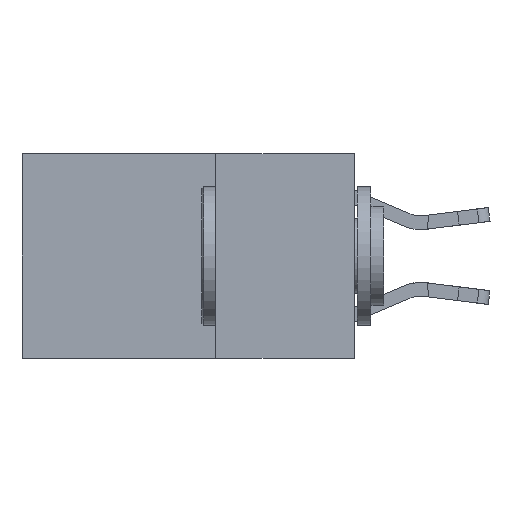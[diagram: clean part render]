
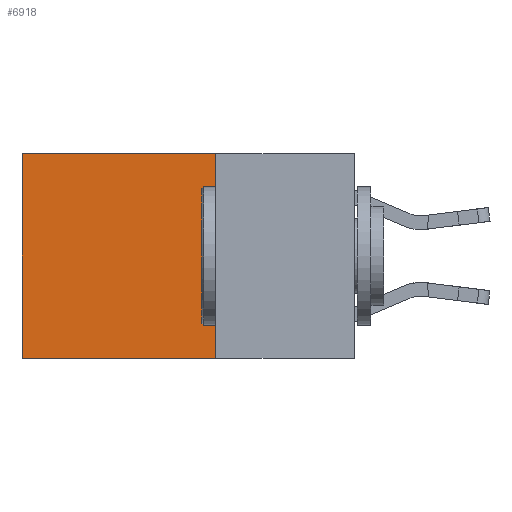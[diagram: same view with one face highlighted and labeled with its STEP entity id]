
A CAD part, left-side view. The second image highlights one B-rep face of the part: STEP entity #6918.
In plain terms, the highlighted planar face has unit normal (-1, 0, 0).
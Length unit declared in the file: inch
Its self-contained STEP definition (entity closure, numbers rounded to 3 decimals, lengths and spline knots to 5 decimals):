
#25 = LINE ( 'NONE', #16670, #8484 ) ;
#30 = VERTEX_POINT ( 'NONE', #15405 ) ;
#818 = AXIS2_PLACEMENT_3D ( 'NONE', #14815, #3728, #6355 ) ;
#2178 = FACE_OUTER_BOUND ( 'NONE', #3629, .T. ) ;
#3294 = CARTESIAN_POINT ( 'NONE',  ( 0.2625, 0.6, 0. ) ) ;
#3479 = VECTOR ( 'NONE', #13571, 39.37008 ) ;
#3629 = EDGE_LOOP ( 'NONE', ( #8943, #17262, #16679, #10003 ) ) ;
#3728 = DIRECTION ( 'NONE',  ( 1., 0., 0. ) ) ;
#3860 = CARTESIAN_POINT ( 'NONE',  ( 0.2625, 0.25, 0. ) ) ;
#3932 = EDGE_CURVE ( 'NONE', #8075, #30, #25, .T. ) ;
#4221 = DIRECTION ( 'NONE',  ( 0., 0., -1. ) ) ;
#5716 = EDGE_CURVE ( 'NONE', #9379, #9397, #15033, .T. ) ;
#5931 = EDGE_CURVE ( 'NONE', #9379, #8075, #6485, .T. ) ;
#6355 = DIRECTION ( 'NONE',  ( 0., 0., -1. ) ) ;
#6485 = LINE ( 'NONE', #17642, #11206 ) ;
#6918 = ADVANCED_FACE ( 'NONE', ( #2178 ), #17601, .F. ) ;
#7273 = LINE ( 'NONE', #12744, #7653 ) ;
#7653 = VECTOR ( 'NONE', #12839, 39.37008 ) ;
#7852 = DIRECTION ( 'NONE',  ( 0., 1., 0. ) ) ;
#8075 = VERTEX_POINT ( 'NONE', #3294 ) ;
#8484 = VECTOR ( 'NONE', #4221, 39.37008 ) ;
#8943 = ORIENTED_EDGE ( 'NONE', *, *, #3932, .T. ) ;
#9379 = VERTEX_POINT ( 'NONE', #3860 ) ;
#9397 = VERTEX_POINT ( 'NONE', #11341 ) ;
#9933 = EDGE_CURVE ( 'NONE', #9397, #30, #7273, .T. ) ;
#10003 = ORIENTED_EDGE ( 'NONE', *, *, #5931, .T. ) ;
#11206 = VECTOR ( 'NONE', #7852, 39.37008 ) ;
#11341 = CARTESIAN_POINT ( 'NONE',  ( 0.2625, 0.25, -0.37 ) ) ;
#12744 = CARTESIAN_POINT ( 'NONE',  ( 0.2625, 0.25, -0.37 ) ) ;
#12839 = DIRECTION ( 'NONE',  ( 0., 1., 0. ) ) ;
#13571 = DIRECTION ( 'NONE',  ( 0., 0., -1. ) ) ;
#13766 = CARTESIAN_POINT ( 'NONE',  ( 0.2625, 0.25, 0. ) ) ;
#14815 = CARTESIAN_POINT ( 'NONE',  ( 0.2625, 0.25, 0. ) ) ;
#15033 = LINE ( 'NONE', #13766, #3479 ) ;
#15405 = CARTESIAN_POINT ( 'NONE',  ( 0.2625, 0.6, -0.37 ) ) ;
#16670 = CARTESIAN_POINT ( 'NONE',  ( 0.2625, 0.6, 0. ) ) ;
#16679 = ORIENTED_EDGE ( 'NONE', *, *, #5716, .F. ) ;
#17262 = ORIENTED_EDGE ( 'NONE', *, *, #9933, .F. ) ;
#17601 = PLANE ( 'NONE',  #818 ) ;
#17642 = CARTESIAN_POINT ( 'NONE',  ( 0.2625, 0.25, 0. ) ) ;
